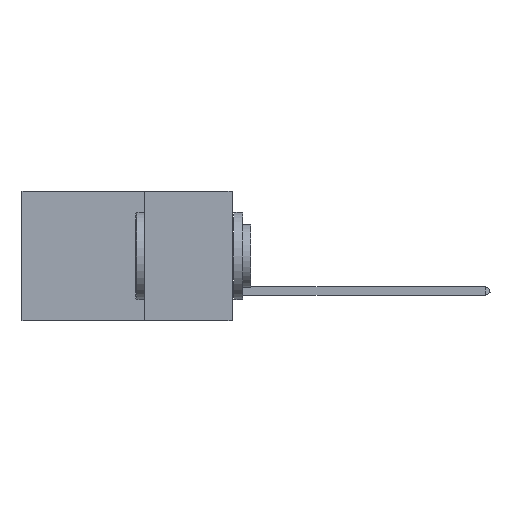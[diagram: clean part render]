
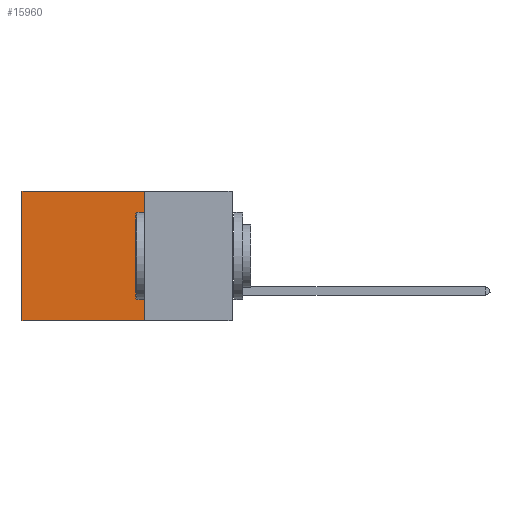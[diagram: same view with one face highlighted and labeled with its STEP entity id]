
A CAD part, left-side view. The second image highlights one B-rep face of the part: STEP entity #15960.
In plain terms, the highlighted planar face has unit normal (-1, 0, 0).
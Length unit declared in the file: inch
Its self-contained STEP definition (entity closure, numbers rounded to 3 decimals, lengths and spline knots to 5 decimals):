
#657 = VERTEX_POINT ( 'NONE', #20873 ) ;
#1823 = CARTESIAN_POINT ( 'NONE',  ( 0.2875, 0.25, -0.37 ) ) ;
#2041 = VECTOR ( 'NONE', #16444, 39.37008 ) ;
#2411 = CARTESIAN_POINT ( 'NONE',  ( 0.2875, 0.25, 0. ) ) ;
#3023 = ORIENTED_EDGE ( 'NONE', *, *, #22549, .T. ) ;
#3169 = CARTESIAN_POINT ( 'NONE',  ( 0.2875, 0.25, 0. ) ) ;
#4497 = ORIENTED_EDGE ( 'NONE', *, *, #15330, .T. ) ;
#5679 = VECTOR ( 'NONE', #22329, 39.37008 ) ;
#6012 = DIRECTION ( 'NONE',  ( 0., 0., -1. ) ) ;
#6302 = DIRECTION ( 'NONE',  ( 0., 1., 0. ) ) ;
#7772 = VECTOR ( 'NONE', #6302, 39.37008 ) ;
#8162 = DIRECTION ( 'NONE',  ( 0., 0., -1. ) ) ;
#8219 = AXIS2_PLACEMENT_3D ( 'NONE', #3169, #15684, #8162 ) ;
#10347 = EDGE_LOOP ( 'NONE', ( #3023, #10759, #20476, #4497 ) ) ;
#10759 = ORIENTED_EDGE ( 'NONE', *, *, #11569, .F. ) ;
#11147 = CARTESIAN_POINT ( 'NONE',  ( 0.2875, 0.6, 0. ) ) ;
#11569 = EDGE_CURVE ( 'NONE', #21410, #657, #15356, .T. ) ;
#13102 = LINE ( 'NONE', #11147, #2041 ) ;
#13189 = FACE_OUTER_BOUND ( 'NONE', #10347, .T. ) ;
#14015 = VERTEX_POINT ( 'NONE', #15657 ) ;
#15168 = LINE ( 'NONE', #2411, #5679 ) ;
#15330 = EDGE_CURVE ( 'NONE', #14015, #17579, #15168, .T. ) ;
#15356 = LINE ( 'NONE', #18953, #7772 ) ;
#15657 = CARTESIAN_POINT ( 'NONE',  ( 0.2875, 0.25, 0. ) ) ;
#15684 = DIRECTION ( 'NONE',  ( 1., 0., 0. ) ) ;
#15960 = ADVANCED_FACE ( 'NONE', ( #13189 ), #22720, .F. ) ;
#16444 = DIRECTION ( 'NONE',  ( 0., 0., -1. ) ) ;
#16699 = CARTESIAN_POINT ( 'NONE',  ( 0.2875, 0.25, 0. ) ) ;
#17579 = VERTEX_POINT ( 'NONE', #17889 ) ;
#17889 = CARTESIAN_POINT ( 'NONE',  ( 0.2875, 0.6, 0. ) ) ;
#18953 = CARTESIAN_POINT ( 'NONE',  ( 0.2875, 0.25, -0.37 ) ) ;
#19839 = LINE ( 'NONE', #16699, #22304 ) ;
#20476 = ORIENTED_EDGE ( 'NONE', *, *, #22006, .F. ) ;
#20873 = CARTESIAN_POINT ( 'NONE',  ( 0.2875, 0.6, -0.37 ) ) ;
#21410 = VERTEX_POINT ( 'NONE', #1823 ) ;
#22006 = EDGE_CURVE ( 'NONE', #14015, #21410, #19839, .T. ) ;
#22304 = VECTOR ( 'NONE', #6012, 39.37008 ) ;
#22329 = DIRECTION ( 'NONE',  ( 0., 1., 0. ) ) ;
#22549 = EDGE_CURVE ( 'NONE', #17579, #657, #13102, .T. ) ;
#22720 = PLANE ( 'NONE',  #8219 ) ;
